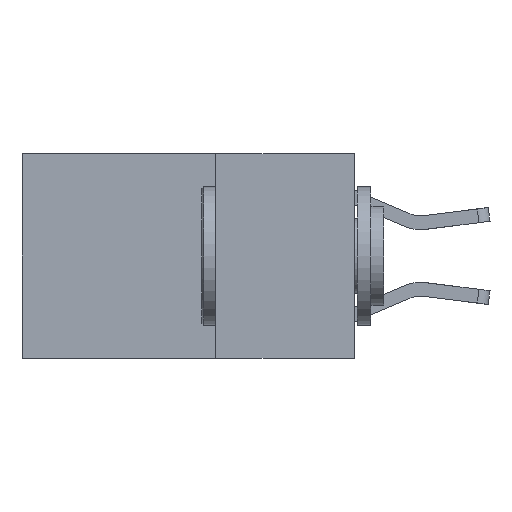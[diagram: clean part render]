
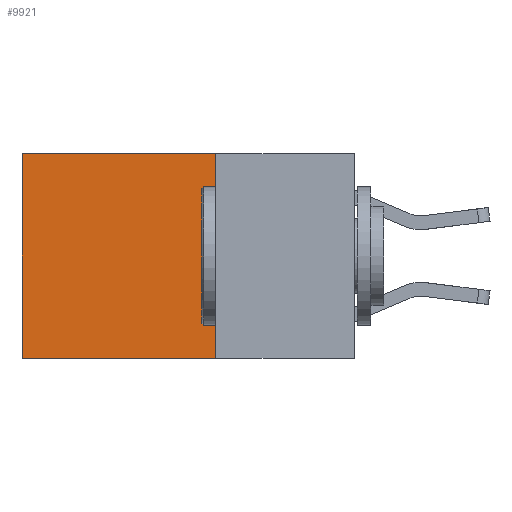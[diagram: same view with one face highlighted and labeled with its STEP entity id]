
A CAD part, left-side view. The second image highlights one B-rep face of the part: STEP entity #9921.
In plain terms, the highlighted planar face has unit normal (-1, 0, 0).
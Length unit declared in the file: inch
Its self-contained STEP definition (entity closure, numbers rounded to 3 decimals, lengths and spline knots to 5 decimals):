
#16 = DIRECTION ( 'NONE',  ( 0., 1., 0. ) ) ;
#631 = EDGE_CURVE ( 'NONE', #4087, #1095, #6316, .T. ) ;
#930 = CARTESIAN_POINT ( 'NONE',  ( 0.2625, 0.6, -0.37 ) ) ;
#1095 = VERTEX_POINT ( 'NONE', #4434 ) ;
#1213 = VECTOR ( 'NONE', #10394, 39.37008 ) ;
#1358 = ORIENTED_EDGE ( 'NONE', *, *, #5843, .T. ) ;
#1515 = CARTESIAN_POINT ( 'NONE',  ( 0.2625, 0.6, 0. ) ) ;
#1519 = VERTEX_POINT ( 'NONE', #930 ) ;
#1714 = CARTESIAN_POINT ( 'NONE',  ( 0.2625, 0.25, 0. ) ) ;
#1876 = VECTOR ( 'NONE', #11746, 39.37008 ) ;
#2480 = VECTOR ( 'NONE', #16, 39.37008 ) ;
#2644 = CARTESIAN_POINT ( 'NONE',  ( 0.2625, 0.25, -0.37 ) ) ;
#3499 = EDGE_LOOP ( 'NONE', ( #6891, #4530, #6576, #1358 ) ) ;
#3583 = VERTEX_POINT ( 'NONE', #3701 ) ;
#3701 = CARTESIAN_POINT ( 'NONE',  ( 0.2625, 0.6, 0. ) ) ;
#3859 = LINE ( 'NONE', #1714, #2480 ) ;
#4087 = VERTEX_POINT ( 'NONE', #9190 ) ;
#4197 = PLANE ( 'NONE',  #12211 ) ;
#4356 = LINE ( 'NONE', #1515, #1876 ) ;
#4416 = EDGE_CURVE ( 'NONE', #3583, #1519, #4356, .T. ) ;
#4434 = CARTESIAN_POINT ( 'NONE',  ( 0.2625, 0.25, -0.37 ) ) ;
#4530 = ORIENTED_EDGE ( 'NONE', *, *, #10084, .F. ) ;
#5843 = EDGE_CURVE ( 'NONE', #4087, #3583, #3859, .T. ) ;
#6120 = DIRECTION ( 'NONE',  ( 0., 0., -1. ) ) ;
#6316 = LINE ( 'NONE', #9582, #1213 ) ;
#6576 = ORIENTED_EDGE ( 'NONE', *, *, #631, .F. ) ;
#6891 = ORIENTED_EDGE ( 'NONE', *, *, #4416, .T. ) ;
#7668 = VECTOR ( 'NONE', #10212, 39.37008 ) ;
#7976 = CARTESIAN_POINT ( 'NONE',  ( 0.2625, 0.25, 0. ) ) ;
#8218 = LINE ( 'NONE', #2644, #7668 ) ;
#8912 = FACE_OUTER_BOUND ( 'NONE', #3499, .T. ) ;
#9190 = CARTESIAN_POINT ( 'NONE',  ( 0.2625, 0.25, 0. ) ) ;
#9582 = CARTESIAN_POINT ( 'NONE',  ( 0.2625, 0.25, 0. ) ) ;
#9921 = ADVANCED_FACE ( 'NONE', ( #8912 ), #4197, .F. ) ;
#10084 = EDGE_CURVE ( 'NONE', #1095, #1519, #8218, .T. ) ;
#10212 = DIRECTION ( 'NONE',  ( 0., 1., 0. ) ) ;
#10394 = DIRECTION ( 'NONE',  ( 0., 0., -1. ) ) ;
#11746 = DIRECTION ( 'NONE',  ( 0., 0., -1. ) ) ;
#11770 = DIRECTION ( 'NONE',  ( 1., 0., 0. ) ) ;
#12211 = AXIS2_PLACEMENT_3D ( 'NONE', #7976, #11770, #6120 ) ;
